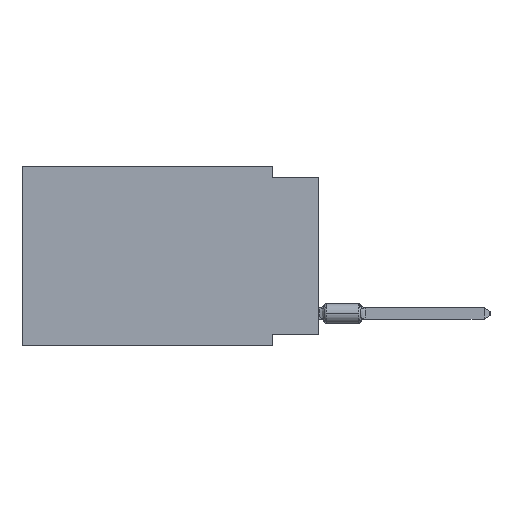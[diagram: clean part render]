
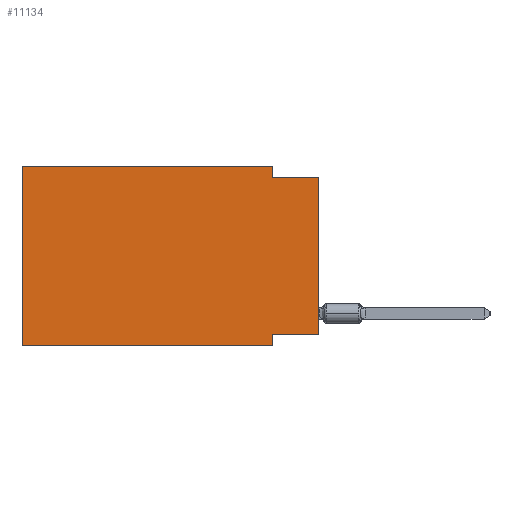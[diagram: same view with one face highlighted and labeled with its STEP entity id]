
A CAD part, left-side view. The second image highlights one B-rep face of the part: STEP entity #11134.
In plain terms, the highlighted planar face has unit normal (-1, 0, 0).
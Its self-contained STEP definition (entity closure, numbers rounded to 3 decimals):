
#2829 = DIRECTION ( 'NONE',  ( 0., 0., -1. ) ) ;
#8069 = VECTOR ( 'NONE', #56922, 1000. ) ;
#8790 = CARTESIAN_POINT ( 'NONE',  ( 0., 2.54, -9.271 ) ) ;
#10090 = LINE ( 'NONE', #41543, #8069 ) ;
#11134 = ADVANCED_FACE ( 'NONE', ( #16639 ), #26901, .F. ) ;
#11215 = DIRECTION ( 'NONE',  ( 0., 1., 0. ) ) ;
#12137 = VERTEX_POINT ( 'NONE', #33410 ) ;
#12296 = VERTEX_POINT ( 'NONE', #67427 ) ;
#12414 = CARTESIAN_POINT ( 'NONE',  ( 0., 2.54, 0. ) ) ;
#13223 = VECTOR ( 'NONE', #2829, 1000. ) ;
#14374 = CARTESIAN_POINT ( 'NONE',  ( 0., 0., -9.271 ) ) ;
#16358 = CARTESIAN_POINT ( 'NONE',  ( 0., 0., -0.635 ) ) ;
#16639 = FACE_OUTER_BOUND ( 'NONE', #22053, .T. ) ;
#16678 = EDGE_CURVE ( 'NONE', #22168, #48999, #21124, .T. ) ;
#17057 = DIRECTION ( 'NONE',  ( 0., 0., 1. ) ) ;
#20083 = LINE ( 'NONE', #20425, #55063 ) ;
#20425 = CARTESIAN_POINT ( 'NONE',  ( 0., 16.383, -9.906 ) ) ;
#20826 = CARTESIAN_POINT ( 'NONE',  ( 0., 16.383, 0. ) ) ;
#21101 = DIRECTION ( 'NONE',  ( 0., -1., 0. ) ) ;
#21124 = LINE ( 'NONE', #57698, #30956 ) ;
#22053 = EDGE_LOOP ( 'NONE', ( #33086, #51844, #36059, #65160, #51346, #59287, #45744, #23651 ) ) ;
#22168 = VERTEX_POINT ( 'NONE', #14374 ) ;
#22450 = DIRECTION ( 'NONE',  ( 0., 0., -1. ) ) ;
#22862 = LINE ( 'NONE', #53965, #28161 ) ;
#23651 = ORIENTED_EDGE ( 'NONE', *, *, #16678, .F. ) ;
#24721 = EDGE_CURVE ( 'NONE', #12137, #44349, #20083, .T. ) ;
#25121 = EDGE_CURVE ( 'NONE', #12296, #26216, #52264, .T. ) ;
#25743 = CARTESIAN_POINT ( 'NONE',  ( 0., 2.54, -0.635 ) ) ;
#26216 = VERTEX_POINT ( 'NONE', #47828 ) ;
#26556 = CARTESIAN_POINT ( 'NONE',  ( 0., 16.383, 0. ) ) ;
#26901 = PLANE ( 'NONE',  #45863 ) ;
#28161 = VECTOR ( 'NONE', #17057, 1000. ) ;
#30133 = EDGE_CURVE ( 'NONE', #22168, #53990, #22862, .T. ) ;
#30956 = VECTOR ( 'NONE', #11215, 1000. ) ;
#32993 = CARTESIAN_POINT ( 'NONE',  ( 0., 0., -0.635 ) ) ;
#33086 = ORIENTED_EDGE ( 'NONE', *, *, #30133, .T. ) ;
#33410 = CARTESIAN_POINT ( 'NONE',  ( 0., 16.383, -9.906 ) ) ;
#34269 = LINE ( 'NONE', #12414, #13223 ) ;
#36059 = ORIENTED_EDGE ( 'NONE', *, *, #66151, .F. ) ;
#36225 = DIRECTION ( 'NONE',  ( 0., -1., 0. ) ) ;
#36849 = EDGE_CURVE ( 'NONE', #58867, #53990, #42335, .T. ) ;
#39147 = CARTESIAN_POINT ( 'NONE',  ( 0., 2.54, -9.906 ) ) ;
#41543 = CARTESIAN_POINT ( 'NONE',  ( 0., 2.54, -9.906 ) ) ;
#42027 = VECTOR ( 'NONE', #36225, 1000. ) ;
#42335 = LINE ( 'NONE', #16358, #58433 ) ;
#42507 = VECTOR ( 'NONE', #51772, 1000. ) ;
#44349 = VERTEX_POINT ( 'NONE', #39147 ) ;
#45744 = ORIENTED_EDGE ( 'NONE', *, *, #58461, .F. ) ;
#45863 = AXIS2_PLACEMENT_3D ( 'NONE', #26556, #57667, #22450 ) ;
#47828 = CARTESIAN_POINT ( 'NONE',  ( 0., 2.54, 0. ) ) ;
#48999 = VERTEX_POINT ( 'NONE', #8790 ) ;
#51346 = ORIENTED_EDGE ( 'NONE', *, *, #64529, .F. ) ;
#51772 = DIRECTION ( 'NONE',  ( 0., 0., 1. ) ) ;
#51844 = ORIENTED_EDGE ( 'NONE', *, *, #36849, .F. ) ;
#52264 = LINE ( 'NONE', #20826, #42027 ) ;
#52934 = DIRECTION ( 'NONE',  ( 0., -1., 0. ) ) ;
#53965 = CARTESIAN_POINT ( 'NONE',  ( 0., 0., 0. ) ) ;
#53990 = VERTEX_POINT ( 'NONE', #32993 ) ;
#55063 = VECTOR ( 'NONE', #21101, 1000. ) ;
#56580 = LINE ( 'NONE', #56913, #42507 ) ;
#56913 = CARTESIAN_POINT ( 'NONE',  ( 0., 16.383, 0. ) ) ;
#56922 = DIRECTION ( 'NONE',  ( 0., 0., -1. ) ) ;
#57667 = DIRECTION ( 'NONE',  ( 1., 0., 0. ) ) ;
#57698 = CARTESIAN_POINT ( 'NONE',  ( 0., 0., -9.271 ) ) ;
#58433 = VECTOR ( 'NONE', #52934, 1000. ) ;
#58461 = EDGE_CURVE ( 'NONE', #48999, #44349, #10090, .T. ) ;
#58867 = VERTEX_POINT ( 'NONE', #25743 ) ;
#59287 = ORIENTED_EDGE ( 'NONE', *, *, #24721, .T. ) ;
#64529 = EDGE_CURVE ( 'NONE', #12137, #12296, #56580, .T. ) ;
#65160 = ORIENTED_EDGE ( 'NONE', *, *, #25121, .F. ) ;
#66151 = EDGE_CURVE ( 'NONE', #26216, #58867, #34269, .T. ) ;
#67427 = CARTESIAN_POINT ( 'NONE',  ( 0., 16.383, 0. ) ) ;
